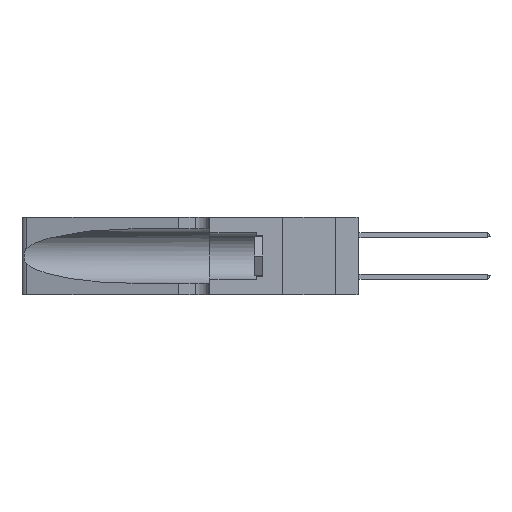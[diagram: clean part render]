
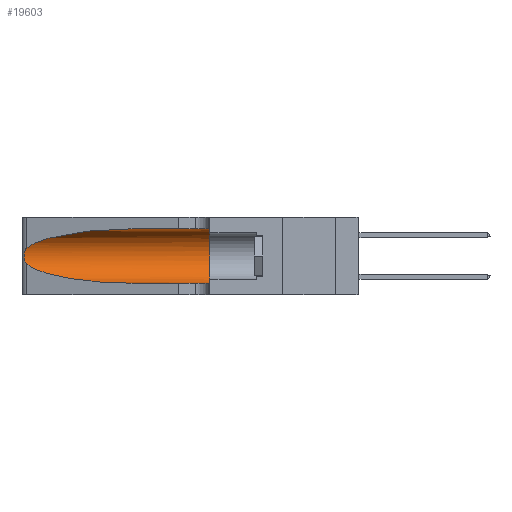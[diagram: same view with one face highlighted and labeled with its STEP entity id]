
A CAD part, left-side view. The second image highlights one B-rep face of the part: STEP entity #19603.
In plain terms, the highlighted cylindrical face has radius 3.308 mm (diameter 6.617 mm), a partial arc.
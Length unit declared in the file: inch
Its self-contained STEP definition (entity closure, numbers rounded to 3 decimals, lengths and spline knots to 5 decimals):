
#426 = CARTESIAN_POINT ( 'NONE',  ( 0.26017, 1.23833, 0.17102 ) ) ;
#1220 = CYLINDRICAL_SURFACE ( 'NONE', #35180, 0.13025 ) ;
#1921 = CARTESIAN_POINT ( 'NONE',  ( 0.1305, 0.72297, 0.05475 ) ) ;
#2163 = FACE_OUTER_BOUND ( 'NONE', #4913, .T. ) ;
#2321 = CARTESIAN_POINT ( 'NONE',  ( 0.1305, 0.35, 0.185 ) ) ;
#2994 = VECTOR ( 'NONE', #4671, 39.37008 ) ;
#3414 = CARTESIAN_POINT ( 'NONE',  ( 0.25789, 1.23486, 0.15765 ) ) ;
#4671 = DIRECTION ( 'NONE',  ( 0., -1., 0. ) ) ;
#4913 = EDGE_LOOP ( 'NONE', ( #31554, #11835, #19215, #17950, #15007, #23289 ) ) ;
#4952 =( BOUNDED_CURVE ( )  B_SPLINE_CURVE ( 3, ( #30449, #7097, #33380, #15904 ),
 .UNSPECIFIED., .F., .F. ) 
 B_SPLINE_CURVE_WITH_KNOTS ( ( 4, 4 ),
 ( 3.44316, 4.71239 ),
 .UNSPECIFIED. ) 
 CURVE ( )  GEOMETRIC_REPRESENTATION_ITEM ( )  RATIONAL_B_SPLINE_CURVE ( ( 1., 0.87, 0.87, 1. ) ) 
 REPRESENTATION_ITEM ( '' )  );
#5294 = DIRECTION ( 'NONE',  ( 0., 0., 1. ) ) ;
#5405 = VECTOR ( 'NONE', #13907, 39.37008 ) ;
#6150 = CARTESIAN_POINT ( 'NONE',  ( 0.25487, 1.22718, 0.22369 ) ) ;
#6283 = CARTESIAN_POINT ( 'NONE',  ( 0.25555, 1.22994, 0.2215 ) ) ;
#6417 = CARTESIAN_POINT ( 'NONE',  ( 0.25555, 1.22993, 0.14849 ) ) ;
#6630 = AXIS2_PLACEMENT_3D ( 'NONE', #2321, #22848, #5294 ) ;
#7097 = CARTESIAN_POINT ( 'NONE',  ( 0.2373, 1.15595, 0.08982 ) ) ;
#8748 = CARTESIAN_POINT ( 'NONE',  ( 0.1305, 1.61858, 0.185 ) ) ;
#10562 = VERTEX_POINT ( 'NONE', #28459 ) ;
#10839 = LINE ( 'NONE', #36695, #2994 ) ;
#10997 = CARTESIAN_POINT ( 'NONE',  ( 0.1305, 1.61858, 0.05475 ) ) ;
#11835 = ORIENTED_EDGE ( 'NONE', *, *, #22937, .T. ) ;
#12177 = CARTESIAN_POINT ( 'NONE',  ( 0.25787, 1.23484, 0.2124 ) ) ;
#13907 = DIRECTION ( 'NONE',  ( 0., -1., 0. ) ) ;
#14574 =( BOUNDED_CURVE ( )  B_SPLINE_CURVE ( 3, ( #23803, #15099, #35480, #18057 ),
 .UNSPECIFIED., .F., .F. ) 
 B_SPLINE_CURVE_WITH_KNOTS ( ( 4, 4 ),
 ( 1.5708, 2.84003 ),
 .UNSPECIFIED. ) 
 CURVE ( )  GEOMETRIC_REPRESENTATION_ITEM ( )  RATIONAL_B_SPLINE_CURVE ( ( 1., 0.87, 0.87, 1. ) ) 
 REPRESENTATION_ITEM ( '' )  );
#15007 = ORIENTED_EDGE ( 'NONE', *, *, #22027, .F. ) ;
#15098 = CARTESIAN_POINT ( 'NONE',  ( 0.26018, 1.23835, 0.19895 ) ) ;
#15099 = CARTESIAN_POINT ( 'NONE',  ( 0.18966, 0.96281, 0.31525 ) ) ;
#15610 = EDGE_CURVE ( 'NONE', #26769, #23252, #14574, .T. ) ;
#15904 = CARTESIAN_POINT ( 'NONE',  ( 0.1305, 0.72297, 0.05475 ) ) ;
#17950 = ORIENTED_EDGE ( 'NONE', *, *, #34674, .T. ) ;
#18055 = CARTESIAN_POINT ( 'NONE',  ( 0.26075, 1.23896, 0.178 ) ) ;
#18057 = CARTESIAN_POINT ( 'NONE',  ( 0.25487, 1.22718, 0.22369 ) ) ;
#19215 = ORIENTED_EDGE ( 'NONE', *, *, #33313, .T. ) ;
#19324 = CARTESIAN_POINT ( 'NONE',  ( 0.25487, 1.22718, 0.22369 ) ) ;
#19603 = ADVANCED_FACE ( 'NONE', ( #2163 ), #1220, .F. ) ;
#20989 = CARTESIAN_POINT ( 'NONE',  ( 0.25856, 1.23593, 0.16098 ) ) ;
#21005 = CARTESIAN_POINT ( 'NONE',  ( 0.1305, 0.35, 0.05475 ) ) ;
#22027 = EDGE_CURVE ( 'NONE', #33199, #28195, #24120, .T. ) ;
#22848 = DIRECTION ( 'NONE',  ( 0., 1., 0. ) ) ;
#22937 = EDGE_CURVE ( 'NONE', #23252, #10562, #32129, .T. ) ;
#23252 = VERTEX_POINT ( 'NONE', #19324 ) ;
#23289 = ORIENTED_EDGE ( 'NONE', *, *, #30845, .F. ) ;
#23803 = CARTESIAN_POINT ( 'NONE',  ( 0.1305, 0.72297, 0.31525 ) ) ;
#23920 = CARTESIAN_POINT ( 'NONE',  ( 0.25639, 1.23186, 0.15144 ) ) ;
#24120 = CIRCLE ( 'NONE', #6630, 0.13025 ) ;
#24467 = CARTESIAN_POINT ( 'NONE',  ( 0.1305, 0.72297, 0.31525 ) ) ;
#26769 = VERTEX_POINT ( 'NONE', #24467 ) ;
#26861 = CARTESIAN_POINT ( 'NONE',  ( 0.25487, 1.22718, 0.14631 ) ) ;
#27035 = CARTESIAN_POINT ( 'NONE',  ( 0.1305, 0.35, 0.31525 ) ) ;
#28195 = VERTEX_POINT ( 'NONE', #21005 ) ;
#28459 = CARTESIAN_POINT ( 'NONE',  ( 0.25487, 1.22718, 0.14631 ) ) ;
#28740 = LINE ( 'NONE', #10997, #5405 ) ;
#29168 = DIRECTION ( 'NONE',  ( 0., -1., 0. ) ) ;
#29660 = CARTESIAN_POINT ( 'NONE',  ( 0.25639, 1.23184, 0.21858 ) ) ;
#30449 = CARTESIAN_POINT ( 'NONE',  ( 0.25487, 1.22718, 0.14631 ) ) ;
#30845 = EDGE_CURVE ( 'NONE', #26769, #33199, #10839, .T. ) ;
#31554 = ORIENTED_EDGE ( 'NONE', *, *, #15610, .T. ) ;
#32100 = DIRECTION ( 'NONE',  ( 0., 0., -1. ) ) ;
#32129 = B_SPLINE_CURVE_WITH_KNOTS ( 'NONE', 3,
 ( #6150, #6283, #29660, #12177, #32576, #15098, #35479, #18055, #426, #20989, #3414, #23920, #6417, #26861 ),
 .UNSPECIFIED., .F., .F.,
 ( 4, 2, 2, 2, 2, 2, 4 ),
 ( 0., 0.00027, 0.00053, 0.00107, 0.0016, 0.00187, 0.00214 ),
 .UNSPECIFIED. ) ;
#32576 = CARTESIAN_POINT ( 'NONE',  ( 0.25854, 1.2359, 0.20912 ) ) ;
#33199 = VERTEX_POINT ( 'NONE', #27035 ) ;
#33313 = EDGE_CURVE ( 'NONE', #10562, #36519, #4952, .T. ) ;
#33380 = CARTESIAN_POINT ( 'NONE',  ( 0.18966, 0.96281, 0.05475 ) ) ;
#34674 = EDGE_CURVE ( 'NONE', #36519, #28195, #28740, .T. ) ;
#35180 = AXIS2_PLACEMENT_3D ( 'NONE', #8748, #29168, #32100 ) ;
#35479 = CARTESIAN_POINT ( 'NONE',  ( 0.26075, 1.23896, 0.19203 ) ) ;
#35480 = CARTESIAN_POINT ( 'NONE',  ( 0.2373, 1.15595, 0.28018 ) ) ;
#36519 = VERTEX_POINT ( 'NONE', #1921 ) ;
#36695 = CARTESIAN_POINT ( 'NONE',  ( 0.1305, 1.61858, 0.31525 ) ) ;
